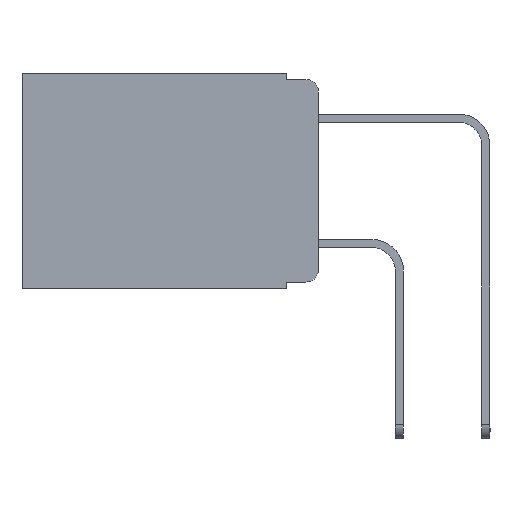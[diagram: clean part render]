
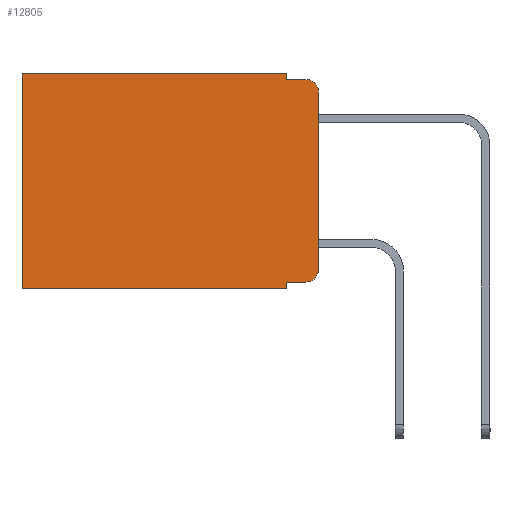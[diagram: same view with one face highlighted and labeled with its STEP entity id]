
A CAD part, left-side view. The second image highlights one B-rep face of the part: STEP entity #12805.
In plain terms, the highlighted planar face has unit normal (-1, 0, 0).
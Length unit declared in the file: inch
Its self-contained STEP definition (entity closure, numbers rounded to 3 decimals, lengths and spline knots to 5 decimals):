
#379 = ORIENTED_EDGE ( 'NONE', *, *, #5634, .F. ) ;
#429 = VERTEX_POINT ( 'NONE', #19103 ) ;
#553 = ORIENTED_EDGE ( 'NONE', *, *, #6051, .T. ) ;
#557 = VECTOR ( 'NONE', #10604, 39.37008 ) ;
#750 = DIRECTION ( 'NONE',  ( 1., 0., 0. ) ) ;
#1076 = DIRECTION ( 'NONE',  ( 0., -1., 0. ) ) ;
#3422 = DIRECTION ( 'NONE',  ( 0., 0., -1. ) ) ;
#3454 = VECTOR ( 'NONE', #13277, 39.37008 ) ;
#3881 = FACE_OUTER_BOUND ( 'NONE', #6802, .T. ) ;
#4110 = CARTESIAN_POINT ( 'NONE',  ( 0.298, 0.051, -0.01 ) ) ;
#4164 = CARTESIAN_POINT ( 'NONE',  ( 0.298, 0., 0. ) ) ;
#4302 = EDGE_CURVE ( 'NONE', #8564, #10439, #13041, .T. ) ;
#4358 = LINE ( 'NONE', #4164, #557 ) ;
#4427 = ORIENTED_EDGE ( 'NONE', *, *, #4302, .F. ) ;
#4738 = VERTEX_POINT ( 'NONE', #12611 ) ;
#4757 = DIRECTION ( 'NONE',  ( 0., 0., -1. ) ) ;
#5274 = EDGE_CURVE ( 'NONE', #13430, #10870, #6683, .T. ) ;
#5634 = EDGE_CURVE ( 'NONE', #10866, #10870, #18318, .T. ) ;
#5775 = CIRCLE ( 'NONE', #18507, 0.02 ) ;
#6003 = ORIENTED_EDGE ( 'NONE', *, *, #16851, .F. ) ;
#6051 = EDGE_CURVE ( 'NONE', #8564, #15368, #16453, .T. ) ;
#6480 = CARTESIAN_POINT ( 'NONE',  ( 0.298, 0.473, 0. ) ) ;
#6673 = ORIENTED_EDGE ( 'NONE', *, *, #8264, .F. ) ;
#6683 = CIRCLE ( 'NONE', #16814, 0.02 ) ;
#6802 = EDGE_LOOP ( 'NONE', ( #6003, #7511, #379, #12370, #7552, #10895, #6673, #4427, #553, #9986 ) ) ;
#6945 = CARTESIAN_POINT ( 'NONE',  ( 0.298, 0.051, -0.333 ) ) ;
#7511 = ORIENTED_EDGE ( 'NONE', *, *, #5274, .T. ) ;
#7552 = ORIENTED_EDGE ( 'NONE', *, *, #16569, .T. ) ;
#7780 = CARTESIAN_POINT ( 'NONE',  ( 0.298, 0.02, -0.01 ) ) ;
#7824 = VERTEX_POINT ( 'NONE', #16237 ) ;
#8074 = CARTESIAN_POINT ( 'NONE',  ( 0.298, 0., -0.313 ) ) ;
#8264 = EDGE_CURVE ( 'NONE', #10439, #4738, #17647, .T. ) ;
#8564 = VERTEX_POINT ( 'NONE', #6945 ) ;
#8930 = LINE ( 'NONE', #20063, #12286 ) ;
#9042 = CARTESIAN_POINT ( 'NONE',  ( 0.298, 0.051, -0.343 ) ) ;
#9325 = DIRECTION ( 'NONE',  ( 0., 0., -1. ) ) ;
#9433 = DIRECTION ( 'NONE',  ( -1., 0., 0. ) ) ;
#9980 = CARTESIAN_POINT ( 'NONE',  ( 0.298, 0., -0.343 ) ) ;
#9986 = ORIENTED_EDGE ( 'NONE', *, *, #17455, .T. ) ;
#10123 = CARTESIAN_POINT ( 'NONE',  ( 0.298, 0.02, -0.313 ) ) ;
#10124 = DIRECTION ( 'NONE',  ( 0., 0., -1. ) ) ;
#10439 = VERTEX_POINT ( 'NONE', #9042 ) ;
#10604 = DIRECTION ( 'NONE',  ( 0., 1., 0. ) ) ;
#10866 = VERTEX_POINT ( 'NONE', #16797 ) ;
#10870 = VERTEX_POINT ( 'NONE', #7780 ) ;
#10895 = ORIENTED_EDGE ( 'NONE', *, *, #13306, .T. ) ;
#10978 = CARTESIAN_POINT ( 'NONE',  ( 0.298, 0.02, -0.03 ) ) ;
#11335 = LINE ( 'NONE', #6480, #12129 ) ;
#12129 = VECTOR ( 'NONE', #3422, 39.37008 ) ;
#12286 = VECTOR ( 'NONE', #19765, 39.37008 ) ;
#12370 = ORIENTED_EDGE ( 'NONE', *, *, #17691, .F. ) ;
#12611 = CARTESIAN_POINT ( 'NONE',  ( 0.298, 0.473, -0.343 ) ) ;
#12805 = ADVANCED_FACE ( 'NONE', ( #3881 ), #14721, .F. ) ;
#12975 = VECTOR ( 'NONE', #4757, 39.37008 ) ;
#13041 = LINE ( 'NONE', #14678, #19710 ) ;
#13272 = DIRECTION ( 'NONE',  ( -1., 0., 0. ) ) ;
#13277 = DIRECTION ( 'NONE',  ( 0., -1., 0. ) ) ;
#13306 = EDGE_CURVE ( 'NONE', #429, #4738, #11335, .T. ) ;
#13430 = VERTEX_POINT ( 'NONE', #14048 ) ;
#13628 = VECTOR ( 'NONE', #18861, 39.37008 ) ;
#14048 = CARTESIAN_POINT ( 'NONE',  ( 0.298, 0., -0.03 ) ) ;
#14678 = CARTESIAN_POINT ( 'NONE',  ( 0.298, 0.051, 0. ) ) ;
#14721 = PLANE ( 'NONE',  #17665 ) ;
#15222 = CARTESIAN_POINT ( 'NONE',  ( 0.298, 0.051, -0.333 ) ) ;
#15368 = VERTEX_POINT ( 'NONE', #18265 ) ;
#15501 = CARTESIAN_POINT ( 'NONE',  ( 0.298, 0.051, 0. ) ) ;
#16237 = CARTESIAN_POINT ( 'NONE',  ( 0.298, 0.051, 0. ) ) ;
#16250 = DIRECTION ( 'NONE',  ( 0., 0., -1. ) ) ;
#16447 = CARTESIAN_POINT ( 'NONE',  ( 0.298, 0., 0. ) ) ;
#16453 = LINE ( 'NONE', #15222, #3454 ) ;
#16491 = VECTOR ( 'NONE', #1076, 39.37008 ) ;
#16569 = EDGE_CURVE ( 'NONE', #7824, #429, #4358, .T. ) ;
#16797 = CARTESIAN_POINT ( 'NONE',  ( 0.298, 0.051, -0.01 ) ) ;
#16814 = AXIS2_PLACEMENT_3D ( 'NONE', #10978, #9433, #9325 ) ;
#16851 = EDGE_CURVE ( 'NONE', #13430, #18664, #8930, .T. ) ;
#17038 = LINE ( 'NONE', #15501, #12975 ) ;
#17455 = EDGE_CURVE ( 'NONE', #15368, #18664, #5775, .T. ) ;
#17538 = DIRECTION ( 'NONE',  ( 0., 0., -1. ) ) ;
#17647 = LINE ( 'NONE', #9980, #13628 ) ;
#17665 = AXIS2_PLACEMENT_3D ( 'NONE', #16447, #750, #10124 ) ;
#17691 = EDGE_CURVE ( 'NONE', #7824, #10866, #17038, .T. ) ;
#18265 = CARTESIAN_POINT ( 'NONE',  ( 0.298, 0.02, -0.333 ) ) ;
#18318 = LINE ( 'NONE', #4110, #16491 ) ;
#18507 = AXIS2_PLACEMENT_3D ( 'NONE', #10123, #13272, #16250 ) ;
#18664 = VERTEX_POINT ( 'NONE', #8074 ) ;
#18861 = DIRECTION ( 'NONE',  ( 0., 1., 0. ) ) ;
#19103 = CARTESIAN_POINT ( 'NONE',  ( 0.298, 0.473, 0. ) ) ;
#19710 = VECTOR ( 'NONE', #17538, 39.37008 ) ;
#19765 = DIRECTION ( 'NONE',  ( 0., 0., -1. ) ) ;
#20063 = CARTESIAN_POINT ( 'NONE',  ( 0.298, 0., 0. ) ) ;
